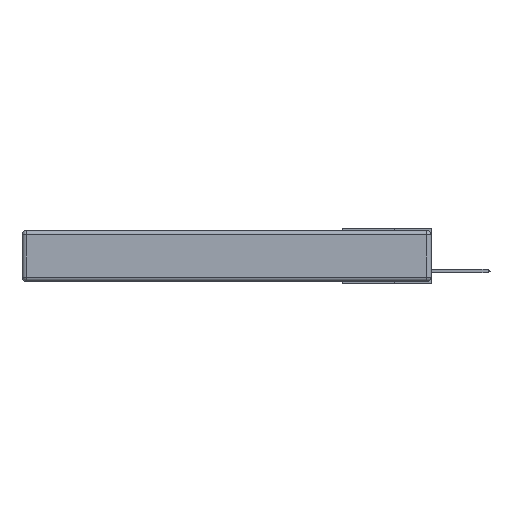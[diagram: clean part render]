
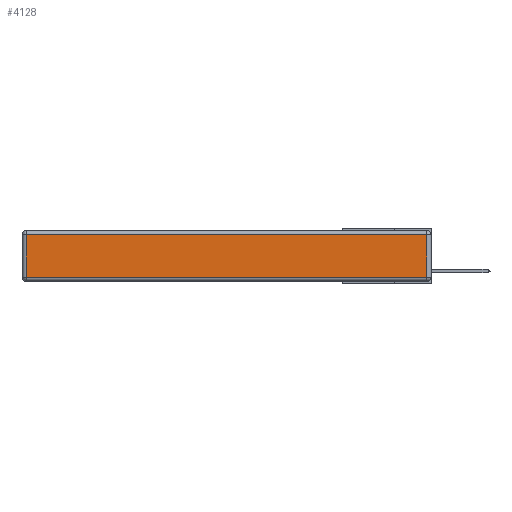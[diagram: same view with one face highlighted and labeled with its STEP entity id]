
A CAD part, left-side view. The second image highlights one B-rep face of the part: STEP entity #4128.
In plain terms, the highlighted planar face has unit normal (-1, 0, 0).
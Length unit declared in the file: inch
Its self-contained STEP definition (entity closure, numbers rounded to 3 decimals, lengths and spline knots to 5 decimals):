
#260 = VECTOR ( 'NONE', #14145, 39.37008 ) ;
#1068 = VERTEX_POINT ( 'NONE', #7500 ) ;
#1077 = EDGE_LOOP ( 'NONE', ( #3276, #16535, #7166, #12335 ) ) ;
#1474 = LINE ( 'NONE', #16747, #260 ) ;
#1645 = VECTOR ( 'NONE', #3092, 39.37008 ) ;
#1683 = VERTEX_POINT ( 'NONE', #10503 ) ;
#1754 = PLANE ( 'NONE',  #9720 ) ;
#2514 = VECTOR ( 'NONE', #13871, 39.37008 ) ;
#2921 = DIRECTION ( 'NONE',  ( 0., -1., 0. ) ) ;
#3092 = DIRECTION ( 'NONE',  ( 0., 1., 0. ) ) ;
#3276 = ORIENTED_EDGE ( 'NONE', *, *, #13527, .T. ) ;
#4128 = ADVANCED_FACE ( 'NONE', ( #13142 ), #1754, .T. ) ;
#4161 = CARTESIAN_POINT ( 'NONE',  ( 0., 2.72, -0.03 ) ) ;
#5542 = DIRECTION ( 'NONE',  ( -1., 0., 0. ) ) ;
#5908 = LINE ( 'NONE', #10534, #8349 ) ;
#6905 = VERTEX_POINT ( 'NONE', #4161 ) ;
#6968 = CARTESIAN_POINT ( 'NONE',  ( 0., 0., -0.343 ) ) ;
#7166 = ORIENTED_EDGE ( 'NONE', *, *, #13771, .T. ) ;
#7500 = CARTESIAN_POINT ( 'NONE',  ( 0., 0.03, -0.03 ) ) ;
#8244 = CARTESIAN_POINT ( 'NONE',  ( 0., 2.75, -0.03 ) ) ;
#8349 = VECTOR ( 'NONE', #2921, 39.37008 ) ;
#9720 = AXIS2_PLACEMENT_3D ( 'NONE', #6968, #5542, #10714 ) ;
#10112 = VERTEX_POINT ( 'NONE', #15422 ) ;
#10503 = CARTESIAN_POINT ( 'NONE',  ( 0., 0.03, -0.313 ) ) ;
#10534 = CARTESIAN_POINT ( 'NONE',  ( 0., 0., -0.313 ) ) ;
#10714 = DIRECTION ( 'NONE',  ( 0., 0., 1. ) ) ;
#11496 = EDGE_CURVE ( 'NONE', #1683, #1068, #11867, .T. ) ;
#11867 = LINE ( 'NONE', #12558, #2514 ) ;
#12335 = ORIENTED_EDGE ( 'NONE', *, *, #12816, .T. ) ;
#12558 = CARTESIAN_POINT ( 'NONE',  ( 0., 0.03, -0.343 ) ) ;
#12816 = EDGE_CURVE ( 'NONE', #6905, #10112, #1474, .T. ) ;
#13142 = FACE_OUTER_BOUND ( 'NONE', #1077, .T. ) ;
#13527 = EDGE_CURVE ( 'NONE', #10112, #1683, #5908, .T. ) ;
#13771 = EDGE_CURVE ( 'NONE', #1068, #6905, #16679, .T. ) ;
#13871 = DIRECTION ( 'NONE',  ( 0., 0., 1. ) ) ;
#14145 = DIRECTION ( 'NONE',  ( 0., 0., -1. ) ) ;
#15422 = CARTESIAN_POINT ( 'NONE',  ( 0., 2.72, -0.313 ) ) ;
#16535 = ORIENTED_EDGE ( 'NONE', *, *, #11496, .T. ) ;
#16679 = LINE ( 'NONE', #8244, #1645 ) ;
#16747 = CARTESIAN_POINT ( 'NONE',  ( 0., 2.72, -0.343 ) ) ;
